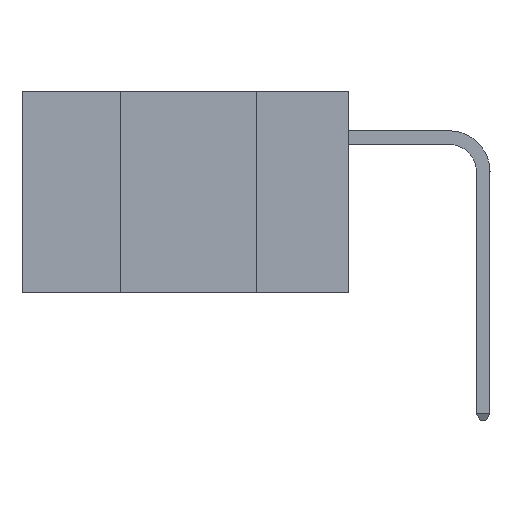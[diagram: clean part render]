
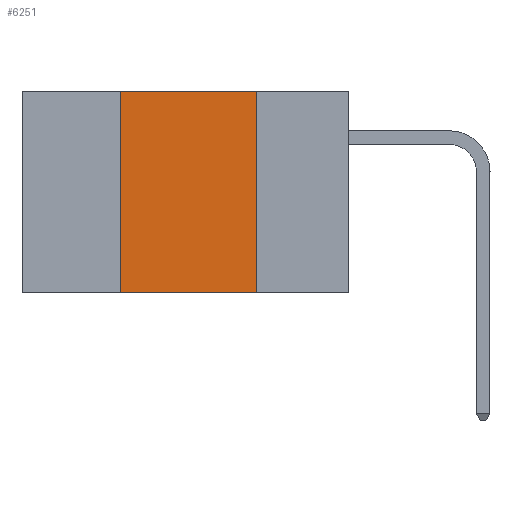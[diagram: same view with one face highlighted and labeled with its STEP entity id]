
A CAD part, left-side view. The second image highlights one B-rep face of the part: STEP entity #6251.
In plain terms, the highlighted planar face has unit normal (-1, 0, 0).
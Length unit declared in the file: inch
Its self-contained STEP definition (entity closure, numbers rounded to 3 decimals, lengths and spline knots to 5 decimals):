
#414 = DIRECTION ( 'NONE',  ( 1., 0., 0. ) ) ;
#618 = CARTESIAN_POINT ( 'NONE',  ( 0., 0.17, 0. ) ) ;
#2678 = EDGE_LOOP ( 'NONE', ( #9657, #18047, #10597, #11278 ) ) ;
#2871 = LINE ( 'NONE', #618, #6170 ) ;
#3589 = LINE ( 'NONE', #13225, #10611 ) ;
#4214 = CARTESIAN_POINT ( 'NONE',  ( 0., 0.42, -0.37 ) ) ;
#4454 = DIRECTION ( 'NONE',  ( 0., 0., 1. ) ) ;
#5697 = VERTEX_POINT ( 'NONE', #10260 ) ;
#6170 = VECTOR ( 'NONE', #11921, 39.37008 ) ;
#6248 = DIRECTION ( 'NONE',  ( 0., -1., 0. ) ) ;
#6251 = ADVANCED_FACE ( 'NONE', ( #17764 ), #7550, .F. ) ;
#7528 = EDGE_CURVE ( 'NONE', #18038, #14025, #14652, .T. ) ;
#7550 = PLANE ( 'NONE',  #15365 ) ;
#9371 = VERTEX_POINT ( 'NONE', #15239 ) ;
#9657 = ORIENTED_EDGE ( 'NONE', *, *, #15893, .F. ) ;
#10260 = CARTESIAN_POINT ( 'NONE',  ( 0., 0.17, 0. ) ) ;
#10377 = DIRECTION ( 'NONE',  ( 0., 0., -1. ) ) ;
#10597 = ORIENTED_EDGE ( 'NONE', *, *, #11263, .F. ) ;
#10611 = VECTOR ( 'NONE', #6248, 39.37008 ) ;
#10965 = VECTOR ( 'NONE', #17697, 39.37008 ) ;
#11263 = EDGE_CURVE ( 'NONE', #18038, #9371, #13493, .T. ) ;
#11278 = ORIENTED_EDGE ( 'NONE', *, *, #7528, .T. ) ;
#11445 = CARTESIAN_POINT ( 'NONE',  ( 0., 0.42, 0. ) ) ;
#11873 = CARTESIAN_POINT ( 'NONE',  ( 0., 0.17, -0.37 ) ) ;
#11921 = DIRECTION ( 'NONE',  ( 0., 0., -1. ) ) ;
#12545 = EDGE_CURVE ( 'NONE', #9371, #5697, #3589, .T. ) ;
#13225 = CARTESIAN_POINT ( 'NONE',  ( 0., 0.6, 0. ) ) ;
#13493 = LINE ( 'NONE', #11445, #17983 ) ;
#14025 = VERTEX_POINT ( 'NONE', #11873 ) ;
#14652 = LINE ( 'NONE', #14958, #10965 ) ;
#14958 = CARTESIAN_POINT ( 'NONE',  ( 0., 0.6, -0.37 ) ) ;
#15239 = CARTESIAN_POINT ( 'NONE',  ( 0., 0.42, 0. ) ) ;
#15365 = AXIS2_PLACEMENT_3D ( 'NONE', #17248, #414, #10377 ) ;
#15893 = EDGE_CURVE ( 'NONE', #5697, #14025, #2871, .T. ) ;
#17248 = CARTESIAN_POINT ( 'NONE',  ( 0., 0.6, 0. ) ) ;
#17697 = DIRECTION ( 'NONE',  ( 0., -1., 0. ) ) ;
#17764 = FACE_OUTER_BOUND ( 'NONE', #2678, .T. ) ;
#17983 = VECTOR ( 'NONE', #4454, 39.37008 ) ;
#18038 = VERTEX_POINT ( 'NONE', #4214 ) ;
#18047 = ORIENTED_EDGE ( 'NONE', *, *, #12545, .F. ) ;
